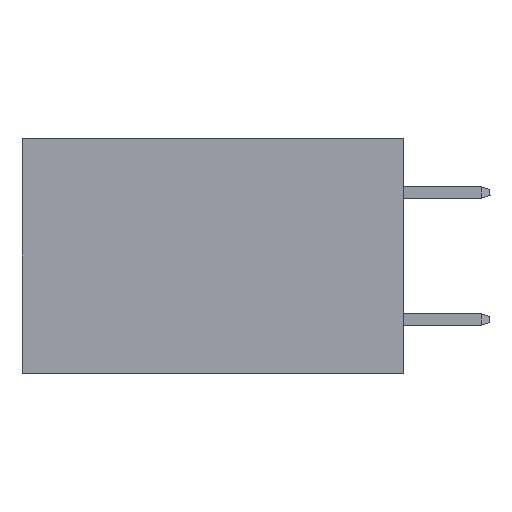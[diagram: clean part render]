
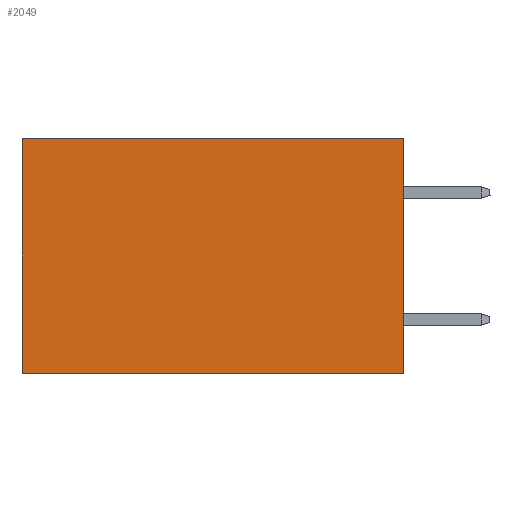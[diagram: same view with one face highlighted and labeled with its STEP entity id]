
A CAD part, left-side view. The second image highlights one B-rep face of the part: STEP entity #2049.
In plain terms, the highlighted planar face has unit normal (-1, 0, 0).
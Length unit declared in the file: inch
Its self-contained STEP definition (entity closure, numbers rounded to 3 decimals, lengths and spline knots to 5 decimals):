
#1305 = DIRECTION ( 'NONE',  ( 0., 0., -1. ) ) ;
#2049 = ADVANCED_FACE ( 'NONE', ( #4475 ), #33482, .F. ) ;
#2526 = CARTESIAN_POINT ( 'NONE',  ( 0.2875, 0., 0. ) ) ;
#3187 = ORIENTED_EDGE ( 'NONE', *, *, #23725, .T. ) ;
#4475 = FACE_OUTER_BOUND ( 'NONE', #34214, .T. ) ;
#7492 = VECTOR ( 'NONE', #25291, 39.37008 ) ;
#7583 = VECTOR ( 'NONE', #24428, 39.37008 ) ;
#8768 = LINE ( 'NONE', #11077, #7583 ) ;
#8891 = EDGE_CURVE ( 'NONE', #21696, #9538, #25115, .T. ) ;
#9538 = VERTEX_POINT ( 'NONE', #18529 ) ;
#10708 = CARTESIAN_POINT ( 'NONE',  ( 0.2875, 0.6, -0.37 ) ) ;
#10942 = CARTESIAN_POINT ( 'NONE',  ( 0.2875, 0.6, 0. ) ) ;
#11077 = CARTESIAN_POINT ( 'NONE',  ( 0.2875, 0., -0.37 ) ) ;
#11118 = VERTEX_POINT ( 'NONE', #10708 ) ;
#11217 = AXIS2_PLACEMENT_3D ( 'NONE', #12218, #15020, #1305 ) ;
#12218 = CARTESIAN_POINT ( 'NONE',  ( 0.2875, 0., 0. ) ) ;
#14566 = CARTESIAN_POINT ( 'NONE',  ( 0.2875, 0., -0.37 ) ) ;
#14901 = ORIENTED_EDGE ( 'NONE', *, *, #24164, .F. ) ;
#15020 = DIRECTION ( 'NONE',  ( 1., 0., 0. ) ) ;
#15118 = VECTOR ( 'NONE', #26824, 39.37008 ) ;
#16467 = EDGE_CURVE ( 'NONE', #21696, #32770, #21527, .T. ) ;
#17251 = ORIENTED_EDGE ( 'NONE', *, *, #16467, .F. ) ;
#18529 = CARTESIAN_POINT ( 'NONE',  ( 0.2875, 0.6, 0. ) ) ;
#21527 = LINE ( 'NONE', #29822, #15118 ) ;
#21696 = VERTEX_POINT ( 'NONE', #2526 ) ;
#23725 = EDGE_CURVE ( 'NONE', #9538, #11118, #27104, .T. ) ;
#24164 = EDGE_CURVE ( 'NONE', #32770, #11118, #8768, .T. ) ;
#24428 = DIRECTION ( 'NONE',  ( 0., 1., 0. ) ) ;
#25115 = LINE ( 'NONE', #33208, #7492 ) ;
#25291 = DIRECTION ( 'NONE',  ( 0., 1., 0. ) ) ;
#26824 = DIRECTION ( 'NONE',  ( 0., 0., -1. ) ) ;
#27104 = LINE ( 'NONE', #10942, #27203 ) ;
#27203 = VECTOR ( 'NONE', #33069, 39.37008 ) ;
#28689 = ORIENTED_EDGE ( 'NONE', *, *, #8891, .T. ) ;
#29822 = CARTESIAN_POINT ( 'NONE',  ( 0.2875, 0., 0. ) ) ;
#32770 = VERTEX_POINT ( 'NONE', #14566 ) ;
#33069 = DIRECTION ( 'NONE',  ( 0., 0., -1. ) ) ;
#33208 = CARTESIAN_POINT ( 'NONE',  ( 0.2875, 0., 0. ) ) ;
#33482 = PLANE ( 'NONE',  #11217 ) ;
#34214 = EDGE_LOOP ( 'NONE', ( #3187, #14901, #17251, #28689 ) ) ;
